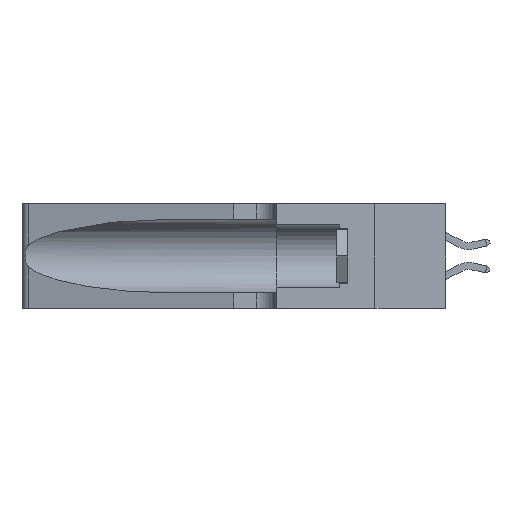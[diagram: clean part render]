
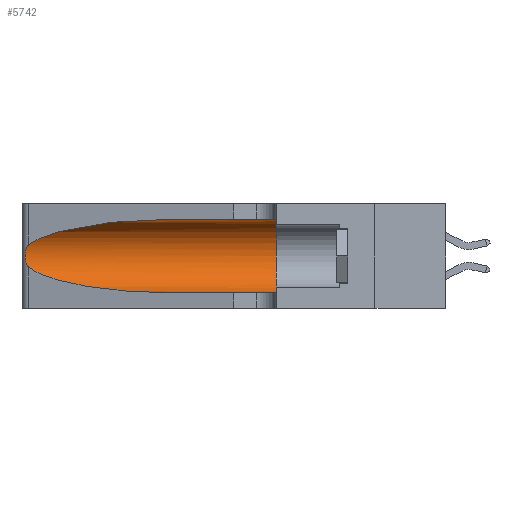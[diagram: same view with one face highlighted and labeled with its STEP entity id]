
A CAD part, left-side view. The second image highlights one B-rep face of the part: STEP entity #5742.
In plain terms, the highlighted cylindrical face has radius 3.308 mm (diameter 6.617 mm), a partial arc.
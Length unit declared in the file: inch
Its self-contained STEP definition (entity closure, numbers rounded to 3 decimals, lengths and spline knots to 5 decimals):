
#281 = VERTEX_POINT ( 'NONE', #2993 ) ;
#412 = DIRECTION ( 'NONE',  ( 0., 0., 1. ) ) ;
#635 = AXIS2_PLACEMENT_3D ( 'NONE', #15232, #7598, #16466 ) ;
#676 = CARTESIAN_POINT ( 'NONE',  ( 0.1305, 0.35, 0.185 ) ) ;
#696 = ORIENTED_EDGE ( 'NONE', *, *, #1654, .F. ) ;
#780 = CARTESIAN_POINT ( 'NONE',  ( 0.25856, 1.23593, 0.16098 ) ) ;
#1016 = DIRECTION ( 'NONE',  ( 0., 1., 0. ) ) ;
#1611 = CIRCLE ( 'NONE', #9657, 0.13025 ) ;
#1654 = EDGE_CURVE ( 'NONE', #8451, #281, #1611, .T. ) ;
#1881 = CARTESIAN_POINT ( 'NONE',  ( 0.25487, 1.22718, 0.14631 ) ) ;
#1928 = EDGE_CURVE ( 'NONE', #4002, #8451, #8699, .T. ) ;
#2093 = CARTESIAN_POINT ( 'NONE',  ( 0.1305, 0.72297, 0.31525 ) ) ;
#2146 = CARTESIAN_POINT ( 'NONE',  ( 0.25555, 1.22994, 0.2215 ) ) ;
#2207 = CARTESIAN_POINT ( 'NONE',  ( 0.25639, 1.23186, 0.15144 ) ) ;
#2391 = ORIENTED_EDGE ( 'NONE', *, *, #9862, .T. ) ;
#2993 = CARTESIAN_POINT ( 'NONE',  ( 0.1305, 0.35, 0.05475 ) ) ;
#3301 = EDGE_CURVE ( 'NONE', #6937, #5450, #6509, .T. ) ;
#3592 = CARTESIAN_POINT ( 'NONE',  ( 0.25487, 1.22718, 0.14631 ) ) ;
#3762 = ORIENTED_EDGE ( 'NONE', *, *, #1928, .F. ) ;
#3851 = ORIENTED_EDGE ( 'NONE', *, *, #10533, .T. ) ;
#4002 = VERTEX_POINT ( 'NONE', #14470 ) ;
#4623 = CARTESIAN_POINT ( 'NONE',  ( 0.25487, 1.22718, 0.22369 ) ) ;
#4827 = CARTESIAN_POINT ( 'NONE',  ( 0.1305, 1.61858, 0.31525 ) ) ;
#4899 = DIRECTION ( 'NONE',  ( 0., -1., 0. ) ) ;
#4909 = CARTESIAN_POINT ( 'NONE',  ( 0.25487, 1.22718, 0.22369 ) ) ;
#4961 = CARTESIAN_POINT ( 'NONE',  ( 0.25639, 1.23184, 0.21858 ) ) ;
#5450 = VERTEX_POINT ( 'NONE', #8283 ) ;
#5742 = ADVANCED_FACE ( 'NONE', ( #12249 ), #11842, .F. ) ;
#5748 = EDGE_CURVE ( 'NONE', #4002, #10080, #8056, .T. ) ;
#6239 = ORIENTED_EDGE ( 'NONE', *, *, #5748, .T. ) ;
#6359 = CARTESIAN_POINT ( 'NONE',  ( 0.25854, 1.2359, 0.20912 ) ) ;
#6509 =( BOUNDED_CURVE ( )  B_SPLINE_CURVE ( 3, ( #10183, #9425, #9540, #8462 ),
 .UNSPECIFIED., .F., .T. ) 
 B_SPLINE_CURVE_WITH_KNOTS ( ( 4, 4 ),
 ( 3.44316, 4.71239 ),
 .UNSPECIFIED. ) 
 CURVE ( )  GEOMETRIC_REPRESENTATION_ITEM ( )  RATIONAL_B_SPLINE_CURVE ( ( 1., 0.87, 0.87, 1. ) ) 
 REPRESENTATION_ITEM ( '' )  );
#6937 = VERTEX_POINT ( 'NONE', #1881 ) ;
#7598 = DIRECTION ( 'NONE',  ( 0., -1., 0. ) ) ;
#7703 = CARTESIAN_POINT ( 'NONE',  ( 0.26075, 1.23896, 0.19203 ) ) ;
#8056 =( BOUNDED_CURVE ( )  B_SPLINE_CURVE ( 3, ( #2093, #10218, #12810, #4909 ),
 .UNSPECIFIED., .F., .F. ) 
 B_SPLINE_CURVE_WITH_KNOTS ( ( 4, 4 ),
 ( 1.5708, 2.84003 ),
 .UNSPECIFIED. ) 
 CURVE ( )  GEOMETRIC_REPRESENTATION_ITEM ( )  RATIONAL_B_SPLINE_CURVE ( ( 1., 0.87, 0.87, 1. ) ) 
 REPRESENTATION_ITEM ( '' )  );
#8283 = CARTESIAN_POINT ( 'NONE',  ( 0.1305, 0.72297, 0.05475 ) ) ;
#8451 = VERTEX_POINT ( 'NONE', #14939 ) ;
#8462 = CARTESIAN_POINT ( 'NONE',  ( 0.1305, 0.72297, 0.05475 ) ) ;
#8699 = LINE ( 'NONE', #4827, #11330 ) ;
#8993 = LINE ( 'NONE', #15823, #11631 ) ;
#9014 = CARTESIAN_POINT ( 'NONE',  ( 0.26017, 1.23833, 0.17102 ) ) ;
#9054 = B_SPLINE_CURVE_WITH_KNOTS ( 'NONE', 3,
 ( #11569, #2146, #4961, #14099, #6359, #15330, #7703, #16565, #9014, #780, #10316, #2207, #11627, #3592 ),
 .UNSPECIFIED., .F., .F.,
 ( 4, 2, 2, 2, 2, 2, 4 ),
 ( 0., 0.00027, 0.00053, 0.00107, 0.0016, 0.00187, 0.00214 ),
 .UNSPECIFIED. ) ;
#9425 = CARTESIAN_POINT ( 'NONE',  ( 0.2373, 1.15595, 0.08982 ) ) ;
#9540 = CARTESIAN_POINT ( 'NONE',  ( 0.18966, 0.96281, 0.05475 ) ) ;
#9657 = AXIS2_PLACEMENT_3D ( 'NONE', #676, #1016, #412 ) ;
#9862 = EDGE_CURVE ( 'NONE', #10080, #6937, #9054, .T. ) ;
#10078 = ORIENTED_EDGE ( 'NONE', *, *, #3301, .T. ) ;
#10080 = VERTEX_POINT ( 'NONE', #4623 ) ;
#10183 = CARTESIAN_POINT ( 'NONE',  ( 0.25487, 1.22718, 0.14631 ) ) ;
#10218 = CARTESIAN_POINT ( 'NONE',  ( 0.18966, 0.96281, 0.31525 ) ) ;
#10278 = EDGE_LOOP ( 'NONE', ( #6239, #2391, #10078, #3851, #696, #3762 ) ) ;
#10316 = CARTESIAN_POINT ( 'NONE',  ( 0.25789, 1.23486, 0.15765 ) ) ;
#10533 = EDGE_CURVE ( 'NONE', #5450, #281, #8993, .T. ) ;
#10836 = DIRECTION ( 'NONE',  ( 0., -1., 0. ) ) ;
#11330 = VECTOR ( 'NONE', #4899, 39.37008 ) ;
#11569 = CARTESIAN_POINT ( 'NONE',  ( 0.25487, 1.22718, 0.22369 ) ) ;
#11627 = CARTESIAN_POINT ( 'NONE',  ( 0.25555, 1.22993, 0.14849 ) ) ;
#11631 = VECTOR ( 'NONE', #10836, 39.37008 ) ;
#11842 = CYLINDRICAL_SURFACE ( 'NONE', #635, 0.13025 ) ;
#12249 = FACE_OUTER_BOUND ( 'NONE', #10278, .T. ) ;
#12810 = CARTESIAN_POINT ( 'NONE',  ( 0.2373, 1.15595, 0.28018 ) ) ;
#14099 = CARTESIAN_POINT ( 'NONE',  ( 0.25787, 1.23484, 0.2124 ) ) ;
#14470 = CARTESIAN_POINT ( 'NONE',  ( 0.1305, 0.72297, 0.31525 ) ) ;
#14939 = CARTESIAN_POINT ( 'NONE',  ( 0.1305, 0.35, 0.31525 ) ) ;
#15232 = CARTESIAN_POINT ( 'NONE',  ( 0.1305, 1.61858, 0.185 ) ) ;
#15330 = CARTESIAN_POINT ( 'NONE',  ( 0.26018, 1.23835, 0.19895 ) ) ;
#15823 = CARTESIAN_POINT ( 'NONE',  ( 0.1305, 1.61858, 0.05475 ) ) ;
#16466 = DIRECTION ( 'NONE',  ( 0., 0., -1. ) ) ;
#16565 = CARTESIAN_POINT ( 'NONE',  ( 0.26075, 1.23896, 0.178 ) ) ;
